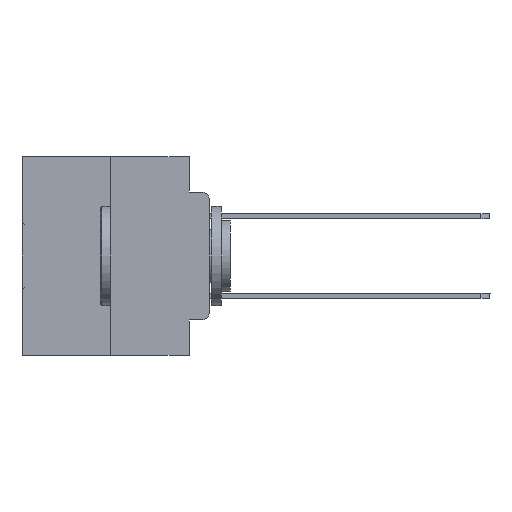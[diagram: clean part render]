
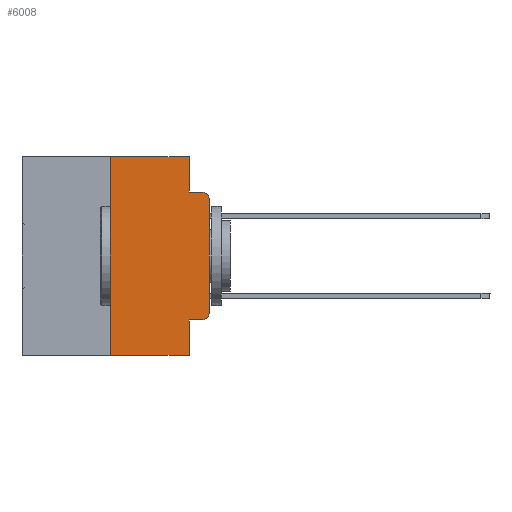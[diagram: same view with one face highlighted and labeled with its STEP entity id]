
A CAD part, left-side view. The second image highlights one B-rep face of the part: STEP entity #6008.
In plain terms, the highlighted planar face has unit normal (-1, 0, 0).
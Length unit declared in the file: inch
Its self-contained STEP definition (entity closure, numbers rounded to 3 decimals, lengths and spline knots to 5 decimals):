
#7 = DIRECTION ( 'NONE',  ( 1., 0., 0. ) ) ;
#236 = CARTESIAN_POINT ( 'NONE',  ( 0., 0.473, 0. ) ) ;
#288 = DIRECTION ( 'NONE',  ( 0., -1., 0. ) ) ;
#423 = DIRECTION ( 'NONE',  ( 0., 0., 1. ) ) ;
#1248 = VERTEX_POINT ( 'NONE', #10187 ) ;
#1292 = DIRECTION ( 'NONE',  ( 0., -1., 0. ) ) ;
#1644 = DIRECTION ( 'NONE',  ( -1., 0., 0. ) ) ;
#2095 = CARTESIAN_POINT ( 'NONE',  ( 0., 0.051, -0.4115 ) ) ;
#2195 = AXIS2_PLACEMENT_3D ( 'NONE', #236, #7, #30809 ) ;
#2380 = EDGE_CURVE ( 'NONE', #18800, #23074, #27577, .T. ) ;
#2653 = CARTESIAN_POINT ( 'NONE',  ( 0., 0.473, -0.5 ) ) ;
#3609 = CARTESIAN_POINT ( 'NONE',  ( 0., 0.02, -0.1085 ) ) ;
#4623 = CIRCLE ( 'NONE', #31576, 0.02 ) ;
#4977 = VECTOR ( 'NONE', #1292, 39.37008 ) ;
#5085 = LINE ( 'NONE', #5911, #26230 ) ;
#5884 = LINE ( 'NONE', #6972, #19830 ) ;
#5911 = CARTESIAN_POINT ( 'NONE',  ( 0., 0.051, 0. ) ) ;
#6008 = ADVANCED_FACE ( 'NONE', ( #20407 ), #12972, .F. ) ;
#6331 = CARTESIAN_POINT ( 'NONE',  ( 0., 0.051, -0.0885 ) ) ;
#6972 = CARTESIAN_POINT ( 'NONE',  ( 0., 0.051, 0. ) ) ;
#6994 = VERTEX_POINT ( 'NONE', #20390 ) ;
#7329 = CARTESIAN_POINT ( 'NONE',  ( 0., 0.02, -0.4115 ) ) ;
#7880 = DIRECTION ( 'NONE',  ( 0., -1., 0. ) ) ;
#8261 = DIRECTION ( 'NONE',  ( 0., 0., -1. ) ) ;
#8272 = VERTEX_POINT ( 'NONE', #25516 ) ;
#8359 = CARTESIAN_POINT ( 'NONE',  ( 0., 0.051, -0.5 ) ) ;
#8394 = CARTESIAN_POINT ( 'NONE',  ( 0., 0., -0.1085 ) ) ;
#8814 = VECTOR ( 'NONE', #288, 39.37008 ) ;
#8819 = DIRECTION ( 'NONE',  ( -1., 0., 0. ) ) ;
#9160 = CARTESIAN_POINT ( 'NONE',  ( 0., 0.051, -0.4115 ) ) ;
#9272 = DIRECTION ( 'NONE',  ( 0., -1., 0. ) ) ;
#9978 = CARTESIAN_POINT ( 'NONE',  ( 0., 0.25, -0.5 ) ) ;
#10154 = EDGE_CURVE ( 'NONE', #1248, #19098, #31296, .T. ) ;
#10187 = CARTESIAN_POINT ( 'NONE',  ( 0., 0.051, -0.0885 ) ) ;
#10333 = VERTEX_POINT ( 'NONE', #7329 ) ;
#10660 = EDGE_CURVE ( 'NONE', #10333, #26264, #26738, .T. ) ;
#10786 = DIRECTION ( 'NONE',  ( 0., 0., 1. ) ) ;
#10868 = LINE ( 'NONE', #15595, #28023 ) ;
#11299 = LINE ( 'NONE', #9160, #30842 ) ;
#11329 = ORIENTED_EDGE ( 'NONE', *, *, #2380, .T. ) ;
#12154 = VERTEX_POINT ( 'NONE', #2095 ) ;
#12972 = PLANE ( 'NONE',  #2195 ) ;
#12990 = LINE ( 'NONE', #28420, #18163 ) ;
#13284 = EDGE_CURVE ( 'NONE', #12154, #23074, #5884, .T. ) ;
#14276 = DIRECTION ( 'NONE',  ( 0., 0., -1. ) ) ;
#15595 = CARTESIAN_POINT ( 'NONE',  ( 0., 0.25, 0. ) ) ;
#16013 = EDGE_CURVE ( 'NONE', #8272, #6994, #20454, .T. ) ;
#16204 = CARTESIAN_POINT ( 'NONE',  ( 0., 0.02, -0.0885 ) ) ;
#16453 = CARTESIAN_POINT ( 'NONE',  ( 0., 0., -0.3915 ) ) ;
#16487 = ORIENTED_EDGE ( 'NONE', *, *, #30447, .T. ) ;
#16816 = CARTESIAN_POINT ( 'NONE',  ( 0., 0.02, -0.3915 ) ) ;
#17211 = EDGE_CURVE ( 'NONE', #28479, #19098, #4623, .T. ) ;
#17658 = ORIENTED_EDGE ( 'NONE', *, *, #32750, .T. ) ;
#17861 = EDGE_CURVE ( 'NONE', #6994, #1248, #5085, .T. ) ;
#18163 = VECTOR ( 'NONE', #423, 39.37008 ) ;
#18465 = VECTOR ( 'NONE', #7880, 39.37008 ) ;
#18800 = VERTEX_POINT ( 'NONE', #9978 ) ;
#19098 = VERTEX_POINT ( 'NONE', #16204 ) ;
#19638 = DIRECTION ( 'NONE',  ( 0., 0., -1. ) ) ;
#19830 = VECTOR ( 'NONE', #19638, 39.37008 ) ;
#20390 = CARTESIAN_POINT ( 'NONE',  ( 0., 0.051, 0. ) ) ;
#20407 = FACE_OUTER_BOUND ( 'NONE', #21854, .T. ) ;
#20428 = EDGE_CURVE ( 'NONE', #18800, #8272, #10868, .T. ) ;
#20454 = LINE ( 'NONE', #23016, #18465 ) ;
#21720 = ORIENTED_EDGE ( 'NONE', *, *, #17211, .T. ) ;
#21831 = ORIENTED_EDGE ( 'NONE', *, *, #10660, .T. ) ;
#21854 = EDGE_LOOP ( 'NONE', ( #16487, #21720, #26116, #31628, #22453, #30235, #11329, #28783, #17658, #21831 ) ) ;
#22453 = ORIENTED_EDGE ( 'NONE', *, *, #16013, .F. ) ;
#23016 = CARTESIAN_POINT ( 'NONE',  ( 0., 0.473, 0. ) ) ;
#23074 = VERTEX_POINT ( 'NONE', #8359 ) ;
#23676 = DIRECTION ( 'NONE',  ( 0., 0., -1. ) ) ;
#25516 = CARTESIAN_POINT ( 'NONE',  ( 0., 0.25, 0. ) ) ;
#26116 = ORIENTED_EDGE ( 'NONE', *, *, #10154, .F. ) ;
#26230 = VECTOR ( 'NONE', #8261, 39.37008 ) ;
#26264 = VERTEX_POINT ( 'NONE', #16453 ) ;
#26738 = CIRCLE ( 'NONE', #28588, 0.02 ) ;
#27577 = LINE ( 'NONE', #2653, #8814 ) ;
#28023 = VECTOR ( 'NONE', #10786, 39.37008 ) ;
#28420 = CARTESIAN_POINT ( 'NONE',  ( 0., 0., 0. ) ) ;
#28479 = VERTEX_POINT ( 'NONE', #8394 ) ;
#28588 = AXIS2_PLACEMENT_3D ( 'NONE', #16816, #1644, #14276 ) ;
#28783 = ORIENTED_EDGE ( 'NONE', *, *, #13284, .F. ) ;
#30235 = ORIENTED_EDGE ( 'NONE', *, *, #20428, .F. ) ;
#30447 = EDGE_CURVE ( 'NONE', #26264, #28479, #12990, .T. ) ;
#30809 = DIRECTION ( 'NONE',  ( 0., 0., -1. ) ) ;
#30842 = VECTOR ( 'NONE', #9272, 39.37008 ) ;
#31296 = LINE ( 'NONE', #6331, #4977 ) ;
#31576 = AXIS2_PLACEMENT_3D ( 'NONE', #3609, #8819, #23676 ) ;
#31628 = ORIENTED_EDGE ( 'NONE', *, *, #17861, .F. ) ;
#32750 = EDGE_CURVE ( 'NONE', #12154, #10333, #11299, .T. ) ;
